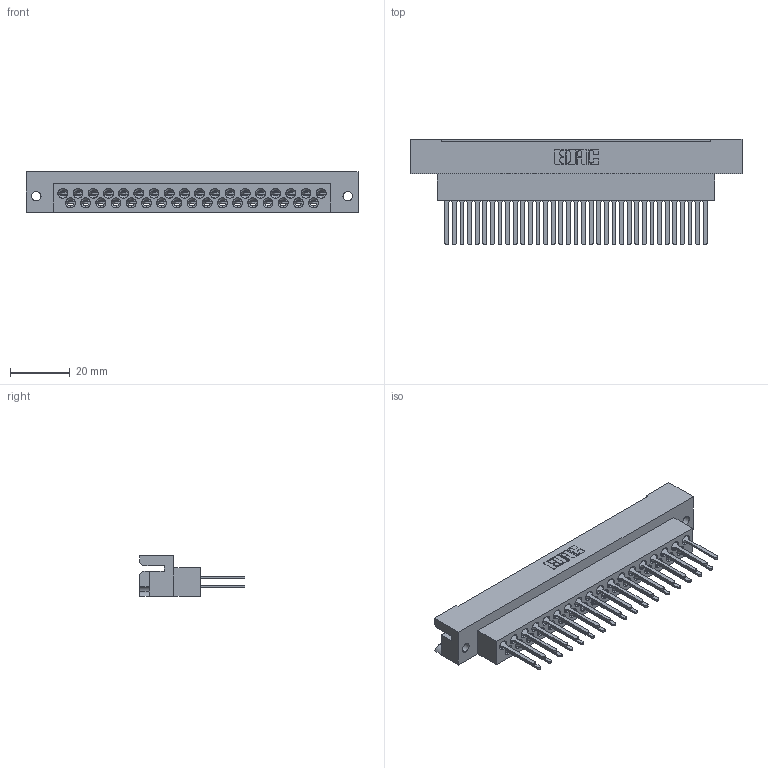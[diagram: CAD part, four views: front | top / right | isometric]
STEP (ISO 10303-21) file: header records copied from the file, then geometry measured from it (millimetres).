
FILE_DESCRIPTION (( 'STEP AP203' ), '1' );
FILE_NAME ('438-035-540-122.STEP', '2020-03-12T20:50:54', ( '' ), ( '' ), 'SwSTEP 2.0', 'SolidWorks 2016', '' );
FILE_SCHEMA (( 'CONFIG_CONTROL_DESIGN' ));
Length unit declared in the file: millimetre
Products named in the file (3): 438-210-001_438-210-035-112; 516-290-001_540; 438-035-540-122
Assembly tree (36 placements, depth 2):
  438-035-540-122
    438-210-001_438-210-035-112
    516-290-001_540  x35
Bounding box: 111 x 35.34 x 13.49 mm (x, y, z)
Volume: 18461.2 mm3; surface area: 23985.1 mm2
Topology: 36 solids, 36 shells, 3586 faces, 10446 edges, 6905 vertices
Faces by surface type: plane 2289, cylinder 960, bspline 232, cone 105
Entity records: 40721 total; most frequent: CARTESIAN_POINT 9395, ORIENTED_EDGE 6748, DIRECTION 5701, EDGE_CURVE 3374, VECTOR 2349, LINE 2349, VERTEX_POINT 2213, AXIS2_PLACEMENT_3D 1676
